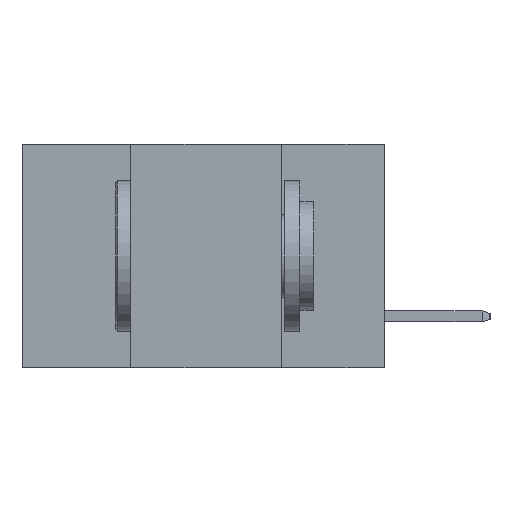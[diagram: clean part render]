
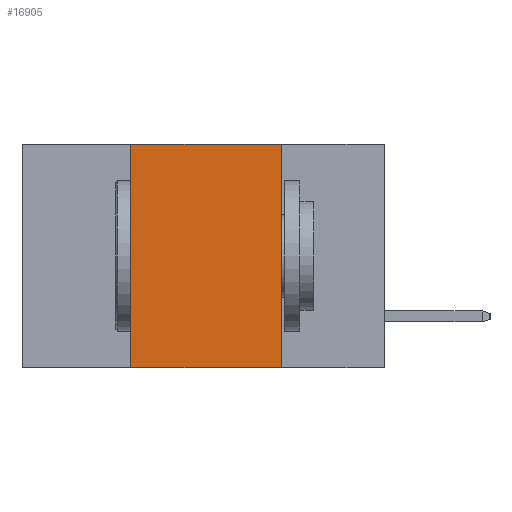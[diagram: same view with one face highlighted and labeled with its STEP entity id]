
A CAD part, left-side view. The second image highlights one B-rep face of the part: STEP entity #16905.
In plain terms, the highlighted planar face has unit normal (-1, 0, 0).
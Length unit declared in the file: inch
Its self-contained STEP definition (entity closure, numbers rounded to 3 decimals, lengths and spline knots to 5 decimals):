
#233 = CARTESIAN_POINT ( 'NONE',  ( 0., 0.17, -0.37 ) ) ;
#1243 = EDGE_CURVE ( 'NONE', #11845, #16671, #6955, .T. ) ;
#1288 = CARTESIAN_POINT ( 'NONE',  ( 0., 0.6, 0. ) ) ;
#2014 = CARTESIAN_POINT ( 'NONE',  ( 0., 0.6, 0. ) ) ;
#2340 = ORIENTED_EDGE ( 'NONE', *, *, #1243, .F. ) ;
#2825 = DIRECTION ( 'NONE',  ( 0., 0., -1. ) ) ;
#3236 = DIRECTION ( 'NONE',  ( 0., 0., -1. ) ) ;
#3260 = CARTESIAN_POINT ( 'NONE',  ( 0., 0.17, 0. ) ) ;
#3356 = VECTOR ( 'NONE', #11136, 39.37008 ) ;
#4319 = PLANE ( 'NONE',  #17807 ) ;
#4843 = EDGE_CURVE ( 'NONE', #9061, #11845, #19356, .T. ) ;
#5754 = FACE_OUTER_BOUND ( 'NONE', #11823, .T. ) ;
#5926 = VECTOR ( 'NONE', #3236, 39.37008 ) ;
#6758 = ORIENTED_EDGE ( 'NONE', *, *, #4843, .F. ) ;
#6859 = CARTESIAN_POINT ( 'NONE',  ( 0., 0.17, 0. ) ) ;
#6873 = EDGE_CURVE ( 'NONE', #16671, #10898, #8494, .T. ) ;
#6955 = LINE ( 'NONE', #2014, #3356 ) ;
#7054 = CARTESIAN_POINT ( 'NONE',  ( 0., 0.6, -0.37 ) ) ;
#7459 = VECTOR ( 'NONE', #13185, 39.37008 ) ;
#7501 = CARTESIAN_POINT ( 'NONE',  ( 0., 0.42, -0.37 ) ) ;
#8494 = LINE ( 'NONE', #3260, #5926 ) ;
#9061 = VERTEX_POINT ( 'NONE', #7501 ) ;
#9492 = ORIENTED_EDGE ( 'NONE', *, *, #6873, .F. ) ;
#10794 = ORIENTED_EDGE ( 'NONE', *, *, #13395, .T. ) ;
#10898 = VERTEX_POINT ( 'NONE', #233 ) ;
#11114 = CARTESIAN_POINT ( 'NONE',  ( 0., 0.42, 0. ) ) ;
#11136 = DIRECTION ( 'NONE',  ( 0., -1., 0. ) ) ;
#11823 = EDGE_LOOP ( 'NONE', ( #9492, #2340, #6758, #10794 ) ) ;
#11845 = VERTEX_POINT ( 'NONE', #11114 ) ;
#11978 = DIRECTION ( 'NONE',  ( 1., 0., 0. ) ) ;
#13185 = DIRECTION ( 'NONE',  ( 0., -1., 0. ) ) ;
#13395 = EDGE_CURVE ( 'NONE', #9061, #10898, #19601, .T. ) ;
#13580 = DIRECTION ( 'NONE',  ( 0., 0., 1. ) ) ;
#16671 = VERTEX_POINT ( 'NONE', #6859 ) ;
#16905 = ADVANCED_FACE ( 'NONE', ( #5754 ), #4319, .F. ) ;
#17617 = CARTESIAN_POINT ( 'NONE',  ( 0., 0.42, 0. ) ) ;
#17807 = AXIS2_PLACEMENT_3D ( 'NONE', #1288, #11978, #2825 ) ;
#18874 = VECTOR ( 'NONE', #13580, 39.37008 ) ;
#19356 = LINE ( 'NONE', #17617, #18874 ) ;
#19601 = LINE ( 'NONE', #7054, #7459 ) ;
